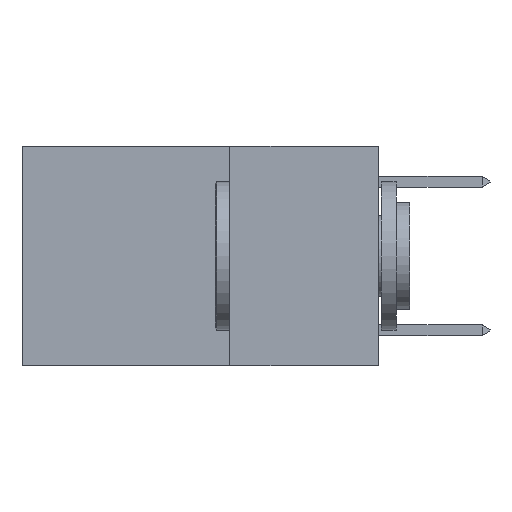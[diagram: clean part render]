
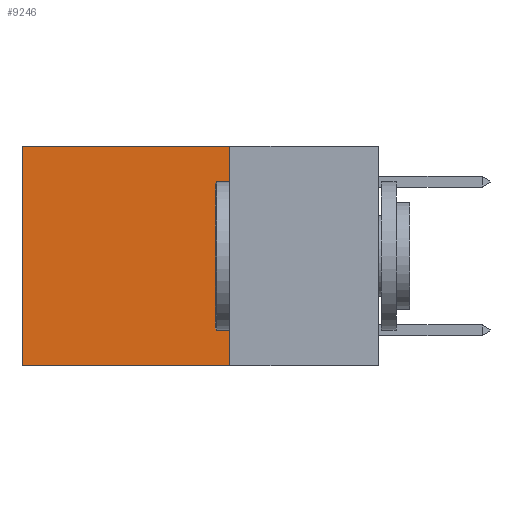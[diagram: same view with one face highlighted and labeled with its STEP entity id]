
A CAD part, left-side view. The second image highlights one B-rep face of the part: STEP entity #9246.
In plain terms, the highlighted planar face has unit normal (-1, 0, 0).
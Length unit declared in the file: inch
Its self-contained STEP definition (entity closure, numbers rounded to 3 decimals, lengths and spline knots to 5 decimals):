
#1020 = VECTOR ( 'NONE', #10655, 39.37008 ) ;
#1214 = CARTESIAN_POINT ( 'NONE',  ( 0.2625, 0.25, 0. ) ) ;
#1298 = LINE ( 'NONE', #10486, #11465 ) ;
#1625 = CARTESIAN_POINT ( 'NONE',  ( 0.2625, 0.6, -0.37 ) ) ;
#1949 = EDGE_LOOP ( 'NONE', ( #2114, #11161, #7297, #11001 ) ) ;
#2006 = LINE ( 'NONE', #1214, #10953 ) ;
#2114 = ORIENTED_EDGE ( 'NONE', *, *, #2751, .T. ) ;
#2180 = CARTESIAN_POINT ( 'NONE',  ( 0.2625, 0.25, -0.37 ) ) ;
#2751 = EDGE_CURVE ( 'NONE', #5795, #5103, #8946, .T. ) ;
#3969 = DIRECTION ( 'NONE',  ( 0., 0., -1. ) ) ;
#4161 = DIRECTION ( 'NONE',  ( 0., 1., 0. ) ) ;
#4592 = EDGE_CURVE ( 'NONE', #5406, #5103, #6101, .T. ) ;
#5103 = VERTEX_POINT ( 'NONE', #1625 ) ;
#5196 = DIRECTION ( 'NONE',  ( 0., 1., 0. ) ) ;
#5406 = VERTEX_POINT ( 'NONE', #8603 ) ;
#5637 = CARTESIAN_POINT ( 'NONE',  ( 0.2625, 0.6, 0. ) ) ;
#5716 = DIRECTION ( 'NONE',  ( 1., 0., 0. ) ) ;
#5795 = VERTEX_POINT ( 'NONE', #5637 ) ;
#6101 = LINE ( 'NONE', #2180, #10149 ) ;
#6832 = CARTESIAN_POINT ( 'NONE',  ( 0.2625, 0.6, 0. ) ) ;
#6985 = AXIS2_PLACEMENT_3D ( 'NONE', #7331, #5716, #8442 ) ;
#7220 = EDGE_CURVE ( 'NONE', #7951, #5795, #1298, .T. ) ;
#7297 = ORIENTED_EDGE ( 'NONE', *, *, #11602, .F. ) ;
#7331 = CARTESIAN_POINT ( 'NONE',  ( 0.2625, 0.25, 0. ) ) ;
#7951 = VERTEX_POINT ( 'NONE', #11867 ) ;
#8442 = DIRECTION ( 'NONE',  ( 0., 0., -1. ) ) ;
#8603 = CARTESIAN_POINT ( 'NONE',  ( 0.2625, 0.25, -0.37 ) ) ;
#8946 = LINE ( 'NONE', #6832, #1020 ) ;
#9246 = ADVANCED_FACE ( 'NONE', ( #9295 ), #11906, .F. ) ;
#9295 = FACE_OUTER_BOUND ( 'NONE', #1949, .T. ) ;
#10149 = VECTOR ( 'NONE', #5196, 39.37008 ) ;
#10486 = CARTESIAN_POINT ( 'NONE',  ( 0.2625, 0.25, 0. ) ) ;
#10655 = DIRECTION ( 'NONE',  ( 0., 0., -1. ) ) ;
#10953 = VECTOR ( 'NONE', #3969, 39.37008 ) ;
#11001 = ORIENTED_EDGE ( 'NONE', *, *, #7220, .T. ) ;
#11161 = ORIENTED_EDGE ( 'NONE', *, *, #4592, .F. ) ;
#11465 = VECTOR ( 'NONE', #4161, 39.37008 ) ;
#11602 = EDGE_CURVE ( 'NONE', #7951, #5406, #2006, .T. ) ;
#11867 = CARTESIAN_POINT ( 'NONE',  ( 0.2625, 0.25, 0. ) ) ;
#11906 = PLANE ( 'NONE',  #6985 ) ;
